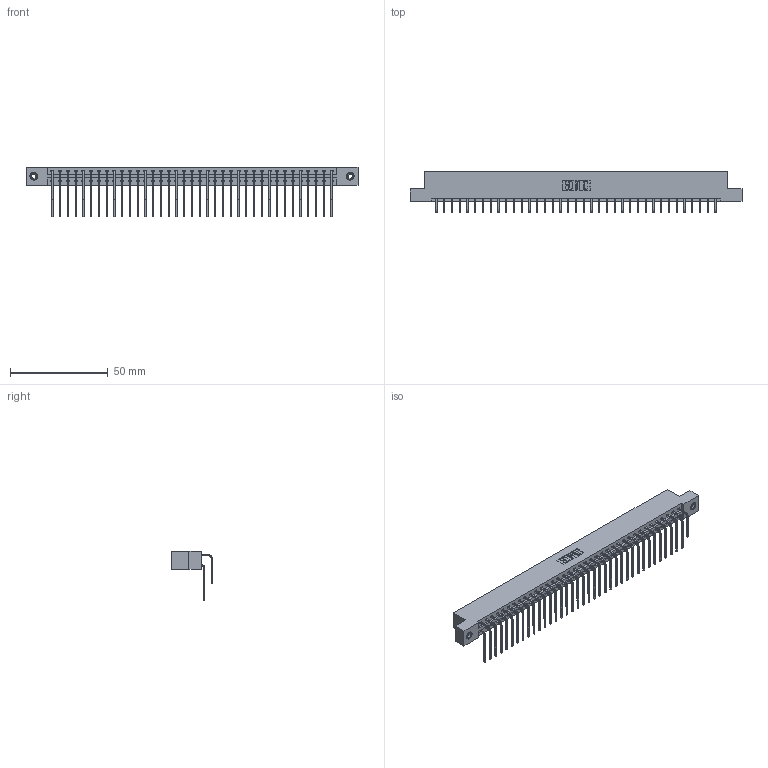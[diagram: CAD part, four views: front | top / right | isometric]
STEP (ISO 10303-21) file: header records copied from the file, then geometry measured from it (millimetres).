
FILE_DESCRIPTION (( 'STEP AP203' ), '1' );
FILE_NAME ('387-074-559-208.STEP', '2018-09-22T20:39:46', ( '' ), ( '' ), 'SwSTEP 2.0', 'SolidWorks 2016', '' );
FILE_SCHEMA (( 'CONFIG_CONTROL_DESIGN' ));
Length unit declared in the file: inch
Products named in the file (5): 345-292-001_558 559 Tail - 1; 345-292-001_559 Tail - 2; 345-250-001_345-250-003-102; 387-074-559-208; 337 Part_Flush Mounting Lugs - 0.156 Dia-TI
Assembly tree (77 placements, depth 2):
  387-074-559-208
    337 Part_Flush Mounting Lugs - 0.156 Dia-TI
    345-292-001_558 559 Tail - 1  x37
    345-292-001_559 Tail - 2  x37
    345-250-001_345-250-003-102  x2
Bounding box: 169.62 x 20.9 x 25.53 mm (x, y, z)
Volume: 18229.8 mm3; surface area: 22727.7 mm2
Topology: 77 solids, 77 shells, 4318 faces, 12805 edges, 8430 vertices
Faces by surface type: plane 3062, cylinder 1240, cone 12, torus 4
Entity records: 32304 total; most frequent: CARTESIAN_POINT 5472, ORIENTED_EDGE 5350, DIRECTION 4677, EDGE_CURVE 2675, LINE 2487, VECTOR 2487, VERTEX_POINT 1776, AXIS2_PLACEMENT_3D 1095
